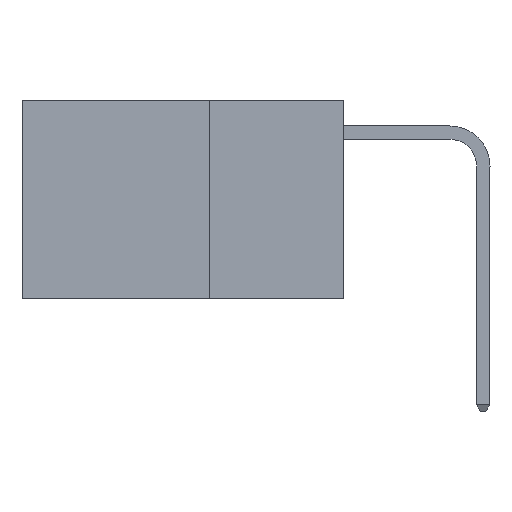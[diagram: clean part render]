
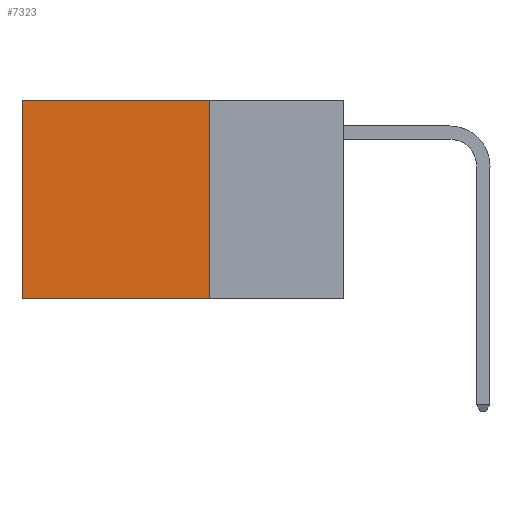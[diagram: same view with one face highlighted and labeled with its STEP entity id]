
A CAD part, left-side view. The second image highlights one B-rep face of the part: STEP entity #7323.
In plain terms, the highlighted planar face has unit normal (-1, 0, 0).
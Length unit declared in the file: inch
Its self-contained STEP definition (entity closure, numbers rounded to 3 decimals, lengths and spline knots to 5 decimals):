
#56 = DIRECTION ( 'NONE',  ( 0., 0., -1. ) ) ;
#280 = CARTESIAN_POINT ( 'NONE',  ( 0.2625, 0.6, -0.37 ) ) ;
#568 = VECTOR ( 'NONE', #6346, 39.37008 ) ;
#590 = DIRECTION ( 'NONE',  ( 0., 1., 0. ) ) ;
#780 = LINE ( 'NONE', #1542, #3879 ) ;
#1417 = CARTESIAN_POINT ( 'NONE',  ( 0.2625, 0.25, 0. ) ) ;
#1542 = CARTESIAN_POINT ( 'NONE',  ( 0.2625, 0.25, 0. ) ) ;
#3415 = ORIENTED_EDGE ( 'NONE', *, *, #4794, .T. ) ;
#3752 = VECTOR ( 'NONE', #56, 39.37008 ) ;
#3879 = VECTOR ( 'NONE', #7151, 39.37008 ) ;
#4032 = CARTESIAN_POINT ( 'NONE',  ( 0.2625, 0.25, 0. ) ) ;
#4498 = VECTOR ( 'NONE', #590, 39.37008 ) ;
#4702 = CARTESIAN_POINT ( 'NONE',  ( 0.2625, 0.6, 0. ) ) ;
#4704 = ORIENTED_EDGE ( 'NONE', *, *, #14259, .F. ) ;
#4794 = EDGE_CURVE ( 'NONE', #8441, #9132, #12472, .T. ) ;
#5244 = CARTESIAN_POINT ( 'NONE',  ( 0.2625, 0.25, -0.37 ) ) ;
#5590 = VERTEX_POINT ( 'NONE', #12538 ) ;
#5621 = ORIENTED_EDGE ( 'NONE', *, *, #10893, .T. ) ;
#5972 = DIRECTION ( 'NONE',  ( 1., 0., 0. ) ) ;
#6346 = DIRECTION ( 'NONE',  ( 0., 1., 0. ) ) ;
#6610 = LINE ( 'NONE', #11795, #568 ) ;
#7151 = DIRECTION ( 'NONE',  ( 0., 0., -1. ) ) ;
#7323 = ADVANCED_FACE ( 'NONE', ( #13400 ), #10379, .F. ) ;
#7419 = LINE ( 'NONE', #4032, #4498 ) ;
#7427 = EDGE_CURVE ( 'NONE', #7443, #9132, #6610, .T. ) ;
#7443 = VERTEX_POINT ( 'NONE', #5244 ) ;
#8441 = VERTEX_POINT ( 'NONE', #12421 ) ;
#8769 = EDGE_LOOP ( 'NONE', ( #3415, #8783, #4704, #5621 ) ) ;
#8783 = ORIENTED_EDGE ( 'NONE', *, *, #7427, .F. ) ;
#9132 = VERTEX_POINT ( 'NONE', #280 ) ;
#10379 = PLANE ( 'NONE',  #11922 ) ;
#10893 = EDGE_CURVE ( 'NONE', #5590, #8441, #7419, .T. ) ;
#11795 = CARTESIAN_POINT ( 'NONE',  ( 0.2625, 0.25, -0.37 ) ) ;
#11922 = AXIS2_PLACEMENT_3D ( 'NONE', #1417, #5972, #13569 ) ;
#12421 = CARTESIAN_POINT ( 'NONE',  ( 0.2625, 0.6, 0. ) ) ;
#12472 = LINE ( 'NONE', #4702, #3752 ) ;
#12538 = CARTESIAN_POINT ( 'NONE',  ( 0.2625, 0.25, 0. ) ) ;
#13400 = FACE_OUTER_BOUND ( 'NONE', #8769, .T. ) ;
#13569 = DIRECTION ( 'NONE',  ( 0., 0., -1. ) ) ;
#14259 = EDGE_CURVE ( 'NONE', #5590, #7443, #780, .T. ) ;
